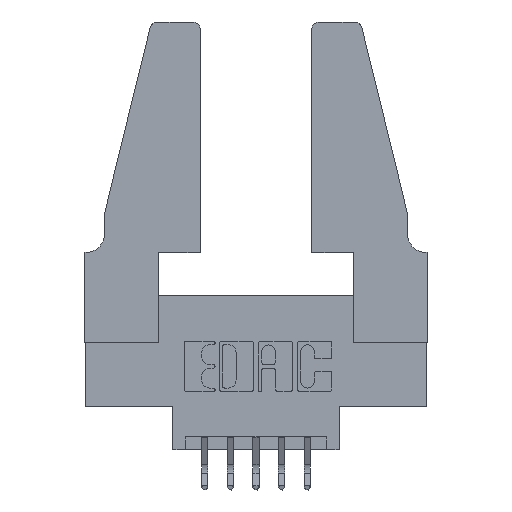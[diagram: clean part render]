
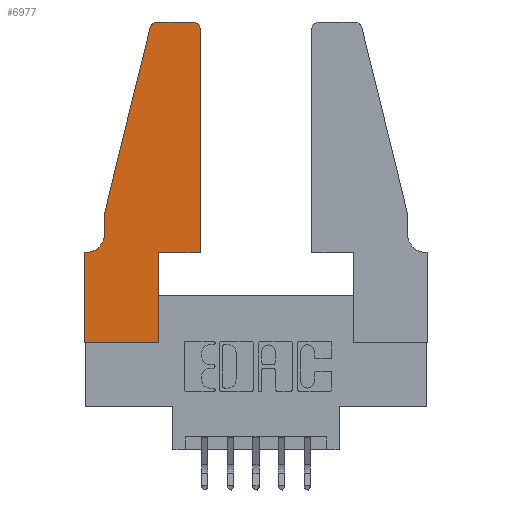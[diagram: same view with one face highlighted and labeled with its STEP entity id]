
A CAD part, top view. The second image highlights one B-rep face of the part: STEP entity #6977.
In plain terms, the highlighted planar face has unit normal (0, 0, 1).
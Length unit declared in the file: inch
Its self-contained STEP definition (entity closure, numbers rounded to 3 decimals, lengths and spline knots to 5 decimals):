
#61 = EDGE_CURVE ( 'NONE', #10669, #2146, #8309, .T. ) ;
#155 = CARTESIAN_POINT ( 'NONE',  ( 0., 0.35, 0.37 ) ) ;
#233 = AXIS2_PLACEMENT_3D ( 'NONE', #7304, #5501, #2034 ) ;
#288 = CIRCLE ( 'NONE', #2218, 0.03 ) ;
#316 = EDGE_CURVE ( 'NONE', #8076, #7705, #288, .T. ) ;
#749 = PLANE ( 'NONE',  #9150 ) ;
#787 = EDGE_CURVE ( 'NONE', #6674, #9130, #2225, .T. ) ;
#908 = CARTESIAN_POINT ( 'NONE',  ( 0.4505, 0.35, 0.37 ) ) ;
#1036 = VECTOR ( 'NONE', #4119, 39.37008 ) ;
#1082 = ORIENTED_EDGE ( 'NONE', *, *, #9830, .T. ) ;
#1179 = LINE ( 'NONE', #5027, #1885 ) ;
#1252 = VECTOR ( 'NONE', #1873, 39.37008 ) ;
#1455 = CARTESIAN_POINT ( 'NONE',  ( 0.0755, 0.35, 0.37 ) ) ;
#1483 = VERTEX_POINT ( 'NONE', #9155 ) ;
#1817 = CARTESIAN_POINT ( 'NONE',  ( 0.0755, 0.5, 0.37 ) ) ;
#1873 = DIRECTION ( 'NONE',  ( 0., 1., 0. ) ) ;
#1885 = VECTOR ( 'NONE', #10168, 39.37008 ) ;
#1903 = EDGE_CURVE ( 'NONE', #7705, #10669, #10898, .T. ) ;
#2034 = DIRECTION ( 'NONE',  ( 1., 0., 0. ) ) ;
#2049 = LINE ( 'NONE', #4352, #7970 ) ;
#2146 = VERTEX_POINT ( 'NONE', #7057 ) ;
#2218 = AXIS2_PLACEMENT_3D ( 'NONE', #4896, #8370, #10152 ) ;
#2225 = LINE ( 'NONE', #908, #1252 ) ;
#2246 = ORIENTED_EDGE ( 'NONE', *, *, #1903, .T. ) ;
#2255 = ORIENTED_EDGE ( 'NONE', *, *, #5041, .T. ) ;
#2281 = DIRECTION ( 'NONE',  ( 0., 1., 0. ) ) ;
#2498 = CIRCLE ( 'NONE', #233, 0.03 ) ;
#2759 = ORIENTED_EDGE ( 'NONE', *, *, #9465, .T. ) ;
#2834 = CARTESIAN_POINT ( 'NONE',  ( 0.0755, 0.5, 0.37 ) ) ;
#2973 = LINE ( 'NONE', #1455, #1036 ) ;
#3292 = CARTESIAN_POINT ( 'NONE',  ( 0., 0., 0.37 ) ) ;
#3421 = DIRECTION ( 'NONE',  ( 0., 0., 1. ) ) ;
#3698 = EDGE_CURVE ( 'NONE', #1483, #8620, #4938, .T. ) ;
#3741 = VERTEX_POINT ( 'NONE', #10824 ) ;
#3905 = EDGE_CURVE ( 'NONE', #8620, #6674, #10157, .T. ) ;
#4079 = DIRECTION ( 'NONE',  ( 1., 0., 0. ) ) ;
#4085 = CARTESIAN_POINT ( 'NONE',  ( 0.284, 1.25, 0.37 ) ) ;
#4119 = DIRECTION ( 'NONE',  ( -1., 0., 0. ) ) ;
#4162 = ORIENTED_EDGE ( 'NONE', *, *, #9333, .T. ) ;
#4200 = DIRECTION ( 'NONE',  ( 1., 0., 0. ) ) ;
#4352 = CARTESIAN_POINT ( 'NONE',  ( 0., 0., 0.37 ) ) ;
#4616 = DIRECTION ( 'NONE',  ( -0.239, -0.971, 0. ) ) ;
#4836 = CARTESIAN_POINT ( 'NONE',  ( 0.4505, 0.35, 0.37 ) ) ;
#4896 = CARTESIAN_POINT ( 'NONE',  ( 0.284, 1.22, 0.37 ) ) ;
#4938 = LINE ( 'NONE', #11081, #9341 ) ;
#4965 = ORIENTED_EDGE ( 'NONE', *, *, #316, .T. ) ;
#5027 = CARTESIAN_POINT ( 'NONE',  ( 0., 0., 0.37 ) ) ;
#5041 = EDGE_CURVE ( 'NONE', #5176, #10016, #2049, .T. ) ;
#5167 = DIRECTION ( 'NONE',  ( -1., 0., 0. ) ) ;
#5176 = VERTEX_POINT ( 'NONE', #155 ) ;
#5185 = CARTESIAN_POINT ( 'NONE',  ( 0.4505, 1.22, 0.37 ) ) ;
#5212 = EDGE_LOOP ( 'NONE', ( #1082, #4965, #2246, #6267, #2759, #11420, #2255, #9535, #9361, #5831, #8937, #4162 ) ) ;
#5301 = VECTOR ( 'NONE', #5167, 39.37008 ) ;
#5349 = DIRECTION ( 'NONE',  ( 0., -1., 0. ) ) ;
#5501 = DIRECTION ( 'NONE',  ( 0., 0., 1. ) ) ;
#5810 = AXIS2_PLACEMENT_3D ( 'NONE', #6716, #11243, #8471 ) ;
#5831 = ORIENTED_EDGE ( 'NONE', *, *, #3905, .T. ) ;
#5989 = CIRCLE ( 'NONE', #5810, 0.07 ) ;
#6180 = EDGE_CURVE ( 'NONE', #8852, #5176, #2973, .T. ) ;
#6206 = VECTOR ( 'NONE', #4079, 39.37008 ) ;
#6267 = ORIENTED_EDGE ( 'NONE', *, *, #61, .T. ) ;
#6546 = VECTOR ( 'NONE', #5349, 39.37008 ) ;
#6586 = CARTESIAN_POINT ( 'NONE',  ( 0.0055, 0.35, 0.37 ) ) ;
#6637 = VECTOR ( 'NONE', #4616, 39.37008 ) ;
#6674 = VERTEX_POINT ( 'NONE', #8906 ) ;
#6716 = CARTESIAN_POINT ( 'NONE',  ( 0.0055, 0.42, 0.37 ) ) ;
#6861 = EDGE_CURVE ( 'NONE', #10016, #1483, #1179, .T. ) ;
#6862 = FACE_OUTER_BOUND ( 'NONE', #5212, .T. ) ;
#6977 = ADVANCED_FACE ( 'NONE', ( #6862 ), #749, .T. ) ;
#7057 = CARTESIAN_POINT ( 'NONE',  ( 0.0755, 0.42, 0.37 ) ) ;
#7304 = CARTESIAN_POINT ( 'NONE',  ( 0.4205, 1.22, 0.37 ) ) ;
#7705 = VERTEX_POINT ( 'NONE', #9531 ) ;
#7970 = VECTOR ( 'NONE', #11298, 39.37008 ) ;
#8076 = VERTEX_POINT ( 'NONE', #4085 ) ;
#8309 = LINE ( 'NONE', #9809, #6546 ) ;
#8370 = DIRECTION ( 'NONE',  ( 0., 0., 1. ) ) ;
#8471 = DIRECTION ( 'NONE',  ( -1., 0., 0. ) ) ;
#8553 = LINE ( 'NONE', #10267, #5301 ) ;
#8620 = VERTEX_POINT ( 'NONE', #10593 ) ;
#8852 = VERTEX_POINT ( 'NONE', #6586 ) ;
#8906 = CARTESIAN_POINT ( 'NONE',  ( 0.4505, 0.35, 0.37 ) ) ;
#8937 = ORIENTED_EDGE ( 'NONE', *, *, #787, .T. ) ;
#9130 = VERTEX_POINT ( 'NONE', #5185 ) ;
#9150 = AXIS2_PLACEMENT_3D ( 'NONE', #10359, #3421, #4200 ) ;
#9155 = CARTESIAN_POINT ( 'NONE',  ( 0.2865, 0., 0.37 ) ) ;
#9333 = EDGE_CURVE ( 'NONE', #9130, #3741, #2498, .T. ) ;
#9341 = VECTOR ( 'NONE', #2281, 39.37008 ) ;
#9361 = ORIENTED_EDGE ( 'NONE', *, *, #3698, .T. ) ;
#9465 = EDGE_CURVE ( 'NONE', #2146, #8852, #5989, .T. ) ;
#9531 = CARTESIAN_POINT ( 'NONE',  ( 0.25487, 1.22718, 0.37 ) ) ;
#9535 = ORIENTED_EDGE ( 'NONE', *, *, #6861, .T. ) ;
#9809 = CARTESIAN_POINT ( 'NONE',  ( 0.0755, 0.5, 0.37 ) ) ;
#9830 = EDGE_CURVE ( 'NONE', #3741, #8076, #8553, .T. ) ;
#10016 = VERTEX_POINT ( 'NONE', #3292 ) ;
#10152 = DIRECTION ( 'NONE',  ( 1., 0., 0. ) ) ;
#10157 = LINE ( 'NONE', #4836, #6206 ) ;
#10168 = DIRECTION ( 'NONE',  ( 1., 0., 0. ) ) ;
#10267 = CARTESIAN_POINT ( 'NONE',  ( 0.2605, 1.25, 0.37 ) ) ;
#10359 = CARTESIAN_POINT ( 'NONE',  ( 0., 0.35, 0.37 ) ) ;
#10593 = CARTESIAN_POINT ( 'NONE',  ( 0.2865, 0.35, 0.37 ) ) ;
#10669 = VERTEX_POINT ( 'NONE', #2834 ) ;
#10824 = CARTESIAN_POINT ( 'NONE',  ( 0.4205, 1.25, 0.37 ) ) ;
#10898 = LINE ( 'NONE', #1817, #6637 ) ;
#11081 = CARTESIAN_POINT ( 'NONE',  ( 0.2865, 0.35, 0.37 ) ) ;
#11243 = DIRECTION ( 'NONE',  ( 0., 0., -1. ) ) ;
#11298 = DIRECTION ( 'NONE',  ( 0., -1., 0. ) ) ;
#11420 = ORIENTED_EDGE ( 'NONE', *, *, #6180, .T. ) ;
